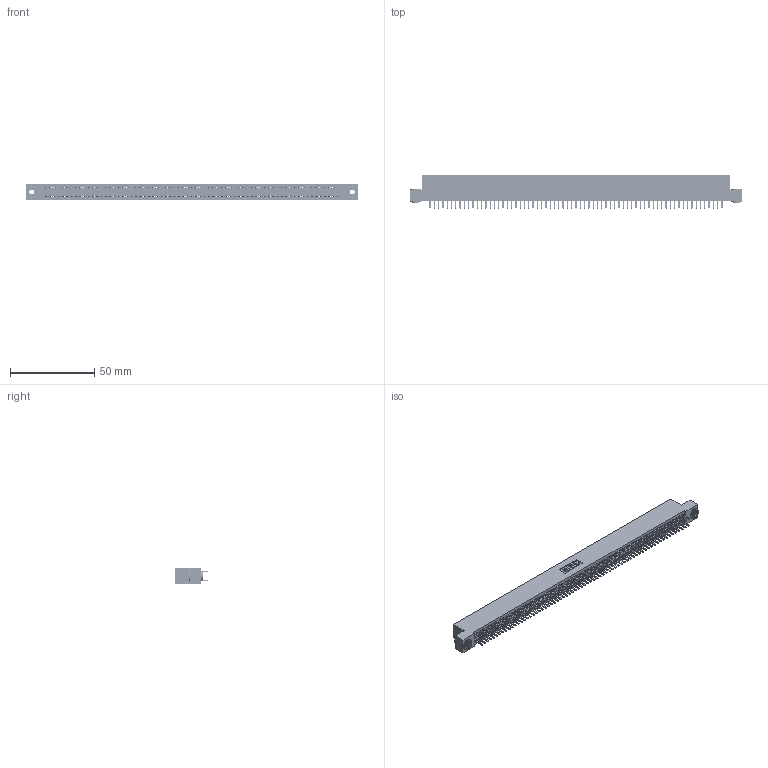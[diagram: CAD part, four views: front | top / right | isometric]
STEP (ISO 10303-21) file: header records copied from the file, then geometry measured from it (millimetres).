
FILE_DESCRIPTION (( 'STEP AP203' ), '1' );
FILE_NAME ('395-138-520-203.STEP', '2019-10-29T18:51:22', ( '' ), ( '' ), 'SwSTEP 2.0', 'SolidWorks 2016', '' );
FILE_SCHEMA (( 'CONFIG_CONTROL_DESIGN' ));
Length unit declared in the file: inch
Products named in the file (4): 345 Part_Flush Mounting Lugs - 0.156 Dia-TH; 345-292-001_345-293-120; 345-250-002_345-250-002-102; 395-138-520-203
Assembly tree (141 placements, depth 2):
  395-138-520-203
    345 Part_Flush Mounting Lugs - 0.156 Dia-TH
    345-292-001_345-293-120  x138
    345-250-002_345-250-002-102  x2
Bounding box: 196.47 x 19.68 x 9.4 mm (x, y, z)
Volume: 19294.5 mm3; surface area: 29119.4 mm2
Topology: 141 solids, 141 shells, 7616 faces, 22083 edges, 14350 vertices
Faces by surface type: plane 4920, cylinder 2688, cone 8
Entity records: 51268 total; most frequent: CARTESIAN_POINT 8555, ORIENTED_EDGE 8470, DIRECTION 7529, EDGE_CURVE 4235, LINE 3799, VECTOR 3799, VERTEX_POINT 2818, AXIS2_PLACEMENT_3D 1865
